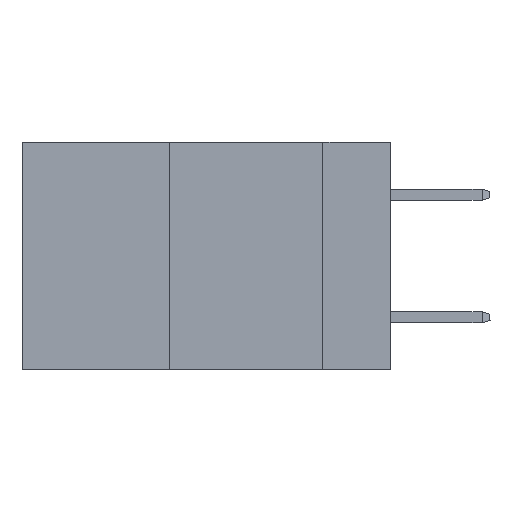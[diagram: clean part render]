
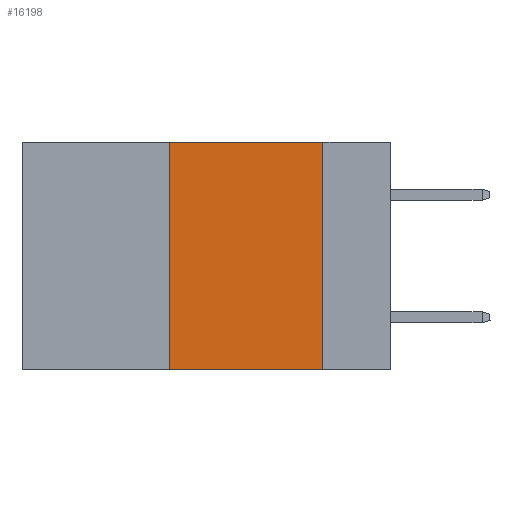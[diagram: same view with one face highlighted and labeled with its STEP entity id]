
A CAD part, left-side view. The second image highlights one B-rep face of the part: STEP entity #16198.
In plain terms, the highlighted planar face has unit normal (-1, 0, 0).
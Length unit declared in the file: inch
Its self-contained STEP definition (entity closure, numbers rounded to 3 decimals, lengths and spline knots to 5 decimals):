
#2 = DIRECTION ( 'NONE',  ( 0., -1., 0. ) ) ;
#410 = DIRECTION ( 'NONE',  ( 0., 0., -1. ) ) ;
#976 = EDGE_CURVE ( 'NONE', #5504, #35542, #7266, .T. ) ;
#2107 = LINE ( 'NONE', #5155, #3393 ) ;
#3181 = VECTOR ( 'NONE', #14982, 39.37008 ) ;
#3393 = VECTOR ( 'NONE', #12714, 39.37008 ) ;
#3450 = VECTOR ( 'NONE', #27619, 39.37008 ) ;
#4594 = ORIENTED_EDGE ( 'NONE', *, *, #15049, .F. ) ;
#5155 = CARTESIAN_POINT ( 'NONE',  ( 0., 0.11, 0. ) ) ;
#5308 = CARTESIAN_POINT ( 'NONE',  ( 0., 0.6, -0.37 ) ) ;
#5504 = VERTEX_POINT ( 'NONE', #9222 ) ;
#7266 = LINE ( 'NONE', #12470, #3181 ) ;
#7952 = CARTESIAN_POINT ( 'NONE',  ( 0., 0.6, 0. ) ) ;
#9221 = AXIS2_PLACEMENT_3D ( 'NONE', #7952, #18910, #410 ) ;
#9222 = CARTESIAN_POINT ( 'NONE',  ( 0., 0.36, -0.37 ) ) ;
#12470 = CARTESIAN_POINT ( 'NONE',  ( 0., 0.36, 0. ) ) ;
#12714 = DIRECTION ( 'NONE',  ( 0., 0., -1. ) ) ;
#14982 = DIRECTION ( 'NONE',  ( 0., 0., 1. ) ) ;
#15049 = EDGE_CURVE ( 'NONE', #25770, #27721, #2107, .T. ) ;
#15879 = EDGE_CURVE ( 'NONE', #5504, #27721, #32657, .T. ) ;
#16198 = ADVANCED_FACE ( 'NONE', ( #27409 ), #24354, .F. ) ;
#16806 = ORIENTED_EDGE ( 'NONE', *, *, #976, .F. ) ;
#17055 = CARTESIAN_POINT ( 'NONE',  ( 0., 0.6, 0. ) ) ;
#18910 = DIRECTION ( 'NONE',  ( 1., 0., 0. ) ) ;
#22727 = ORIENTED_EDGE ( 'NONE', *, *, #31826, .F. ) ;
#24178 = ORIENTED_EDGE ( 'NONE', *, *, #15879, .T. ) ;
#24354 = PLANE ( 'NONE',  #9221 ) ;
#24654 = LINE ( 'NONE', #17055, #25074 ) ;
#25074 = VECTOR ( 'NONE', #2, 39.37008 ) ;
#25770 = VERTEX_POINT ( 'NONE', #33322 ) ;
#27409 = FACE_OUTER_BOUND ( 'NONE', #29300, .T. ) ;
#27619 = DIRECTION ( 'NONE',  ( 0., -1., 0. ) ) ;
#27721 = VERTEX_POINT ( 'NONE', #34087 ) ;
#29300 = EDGE_LOOP ( 'NONE', ( #4594, #22727, #16806, #24178 ) ) ;
#31826 = EDGE_CURVE ( 'NONE', #35542, #25770, #24654, .T. ) ;
#32484 = CARTESIAN_POINT ( 'NONE',  ( 0., 0.36, 0. ) ) ;
#32657 = LINE ( 'NONE', #5308, #3450 ) ;
#33322 = CARTESIAN_POINT ( 'NONE',  ( 0., 0.11, 0. ) ) ;
#34087 = CARTESIAN_POINT ( 'NONE',  ( 0., 0.11, -0.37 ) ) ;
#35542 = VERTEX_POINT ( 'NONE', #32484 ) ;
